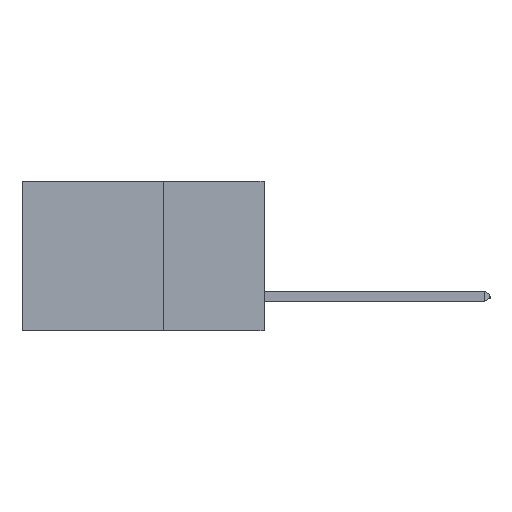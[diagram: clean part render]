
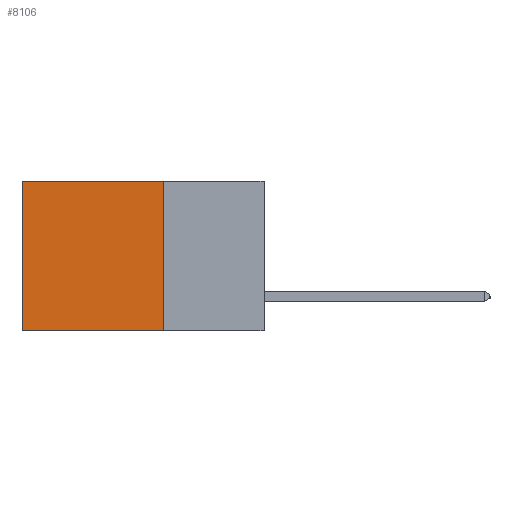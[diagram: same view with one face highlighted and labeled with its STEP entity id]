
A CAD part, left-side view. The second image highlights one B-rep face of the part: STEP entity #8106.
In plain terms, the highlighted planar face has unit normal (-1, 0, 0).
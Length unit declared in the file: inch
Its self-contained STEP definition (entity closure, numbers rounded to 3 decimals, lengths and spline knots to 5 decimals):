
#625 = DIRECTION ( 'NONE',  ( 0., 1., 0. ) ) ;
#646 = DIRECTION ( 'NONE',  ( 0., 0., -1. ) ) ;
#1026 = FACE_OUTER_BOUND ( 'NONE', #15397, .T. ) ;
#1693 = DIRECTION ( 'NONE',  ( 0., 1., 0. ) ) ;
#1993 = CARTESIAN_POINT ( 'NONE',  ( 0.298, 0.25, 0. ) ) ;
#2472 = ORIENTED_EDGE ( 'NONE', *, *, #4550, .F. ) ;
#4114 = CARTESIAN_POINT ( 'NONE',  ( 0.298, 0.6, 0. ) ) ;
#4269 = VERTEX_POINT ( 'NONE', #4114 ) ;
#4279 = VECTOR ( 'NONE', #646, 39.37008 ) ;
#4550 = EDGE_CURVE ( 'NONE', #11743, #10247, #10401, .T. ) ;
#4686 = ORIENTED_EDGE ( 'NONE', *, *, #6476, .T. ) ;
#4808 = CARTESIAN_POINT ( 'NONE',  ( 0.298, 0.6, 0. ) ) ;
#5064 = LINE ( 'NONE', #11716, #4279 ) ;
#5799 = DIRECTION ( 'NONE',  ( 0., 0., -1. ) ) ;
#6358 = CARTESIAN_POINT ( 'NONE',  ( 0.298, 0.25, 0. ) ) ;
#6398 = ORIENTED_EDGE ( 'NONE', *, *, #11704, .F. ) ;
#6476 = EDGE_CURVE ( 'NONE', #9811, #4269, #9979, .T. ) ;
#6881 = CARTESIAN_POINT ( 'NONE',  ( 0.298, 0.25, 0. ) ) ;
#7204 = VECTOR ( 'NONE', #625, 39.37008 ) ;
#8106 = ADVANCED_FACE ( 'NONE', ( #1026 ), #11825, .F. ) ;
#9244 = VECTOR ( 'NONE', #9704, 39.37008 ) ;
#9704 = DIRECTION ( 'NONE',  ( 0., 0., -1. ) ) ;
#9811 = VERTEX_POINT ( 'NONE', #6881 ) ;
#9979 = LINE ( 'NONE', #6358, #12465 ) ;
#10078 = CARTESIAN_POINT ( 'NONE',  ( 0.298, 0.25, -0.37 ) ) ;
#10082 = CARTESIAN_POINT ( 'NONE',  ( 0.298, 0.6, -0.37 ) ) ;
#10247 = VERTEX_POINT ( 'NONE', #10082 ) ;
#10401 = LINE ( 'NONE', #10078, #7204 ) ;
#11704 = EDGE_CURVE ( 'NONE', #9811, #11743, #5064, .T. ) ;
#11716 = CARTESIAN_POINT ( 'NONE',  ( 0.298, 0.25, 0. ) ) ;
#11743 = VERTEX_POINT ( 'NONE', #15380 ) ;
#11825 = PLANE ( 'NONE',  #15530 ) ;
#12453 = LINE ( 'NONE', #4808, #9244 ) ;
#12465 = VECTOR ( 'NONE', #1693, 39.37008 ) ;
#12611 = EDGE_CURVE ( 'NONE', #4269, #10247, #12453, .T. ) ;
#13075 = DIRECTION ( 'NONE',  ( 1., 0., 0. ) ) ;
#14251 = ORIENTED_EDGE ( 'NONE', *, *, #12611, .T. ) ;
#15380 = CARTESIAN_POINT ( 'NONE',  ( 0.298, 0.25, -0.37 ) ) ;
#15397 = EDGE_LOOP ( 'NONE', ( #14251, #2472, #6398, #4686 ) ) ;
#15530 = AXIS2_PLACEMENT_3D ( 'NONE', #1993, #13075, #5799 ) ;
